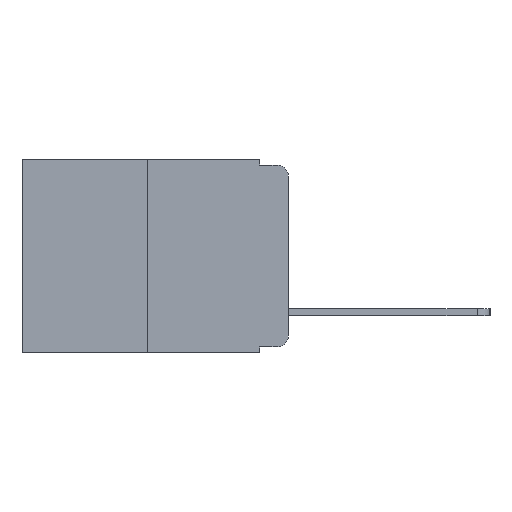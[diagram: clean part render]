
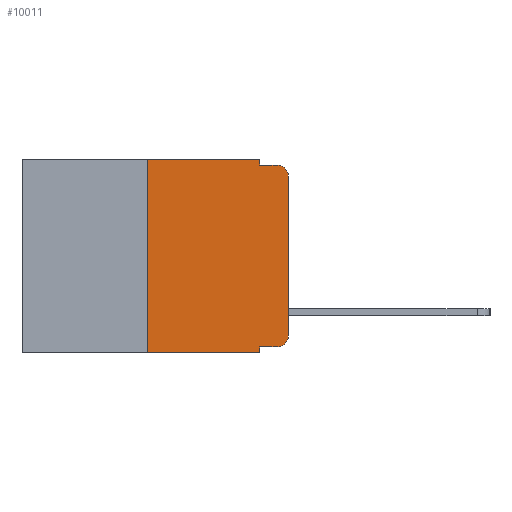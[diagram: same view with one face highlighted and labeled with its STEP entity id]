
A CAD part, left-side view. The second image highlights one B-rep face of the part: STEP entity #10011.
In plain terms, the highlighted planar face has unit normal (-1, 0, 0).
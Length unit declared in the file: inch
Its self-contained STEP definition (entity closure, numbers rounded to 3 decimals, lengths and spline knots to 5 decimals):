
#43 = ORIENTED_EDGE ( 'NONE', *, *, #9116, .T. ) ;
#146 = LINE ( 'NONE', #479, #2923 ) ;
#185 = VERTEX_POINT ( 'NONE', #4592 ) ;
#213 = VECTOR ( 'NONE', #6755, 39.37008 ) ;
#479 = CARTESIAN_POINT ( 'NONE',  ( 0., 0.25, 0. ) ) ;
#668 = CIRCLE ( 'NONE', #10164, 0.02 ) ;
#905 = VERTEX_POINT ( 'NONE', #5850 ) ;
#944 = VECTOR ( 'NONE', #1366, 39.37008 ) ;
#979 = EDGE_CURVE ( 'NONE', #8860, #3241, #3000, .T. ) ;
#1080 = CARTESIAN_POINT ( 'NONE',  ( 0., 0.25, -0.343 ) ) ;
#1091 = VERTEX_POINT ( 'NONE', #9271 ) ;
#1366 = DIRECTION ( 'NONE',  ( 0., -1., 0. ) ) ;
#1451 = EDGE_CURVE ( 'NONE', #7277, #1091, #3312, .T. ) ;
#1468 = DIRECTION ( 'NONE',  ( 0., 0., -1. ) ) ;
#1829 = EDGE_CURVE ( 'NONE', #2506, #3435, #11392, .T. ) ;
#1856 = AXIS2_PLACEMENT_3D ( 'NONE', #3533, #9774, #4496 ) ;
#1991 = CARTESIAN_POINT ( 'NONE',  ( 0., 0.051, 0. ) ) ;
#2491 = ORIENTED_EDGE ( 'NONE', *, *, #979, .T. ) ;
#2506 = VERTEX_POINT ( 'NONE', #7261 ) ;
#2726 = CIRCLE ( 'NONE', #1856, 0.02 ) ;
#2828 = ORIENTED_EDGE ( 'NONE', *, *, #1451, .F. ) ;
#2864 = EDGE_CURVE ( 'NONE', #3435, #905, #668, .T. ) ;
#2923 = VECTOR ( 'NONE', #4551, 39.37008 ) ;
#3000 = LINE ( 'NONE', #10351, #7510 ) ;
#3010 = CARTESIAN_POINT ( 'NONE',  ( 0., 0.051, 0. ) ) ;
#3162 = ORIENTED_EDGE ( 'NONE', *, *, #8479, .F. ) ;
#3241 = VERTEX_POINT ( 'NONE', #6812 ) ;
#3312 = LINE ( 'NONE', #10303, #213 ) ;
#3435 = VERTEX_POINT ( 'NONE', #4904 ) ;
#3533 = CARTESIAN_POINT ( 'NONE',  ( 0., 0.02, -0.03 ) ) ;
#3577 = DIRECTION ( 'NONE',  ( 0., 0., -1. ) ) ;
#3696 = LINE ( 'NONE', #6155, #944 ) ;
#3896 = EDGE_LOOP ( 'NONE', ( #43, #11484, #3162, #5350, #2828, #9760, #2491, #6826, #6556, #6299 ) ) ;
#4271 = VECTOR ( 'NONE', #11627, 39.37008 ) ;
#4496 = DIRECTION ( 'NONE',  ( 0., 0., -1. ) ) ;
#4505 = VECTOR ( 'NONE', #4749, 39.37008 ) ;
#4551 = DIRECTION ( 'NONE',  ( 0., 0., 1. ) ) ;
#4592 = CARTESIAN_POINT ( 'NONE',  ( 0., 0.02, -0.01 ) ) ;
#4749 = DIRECTION ( 'NONE',  ( 0., -1., 0. ) ) ;
#4904 = CARTESIAN_POINT ( 'NONE',  ( 0., 0.02, -0.333 ) ) ;
#4941 = CARTESIAN_POINT ( 'NONE',  ( 0., 0.02, -0.313 ) ) ;
#5346 = PLANE ( 'NONE',  #7872 ) ;
#5350 = ORIENTED_EDGE ( 'NONE', *, *, #11357, .F. ) ;
#5701 = VECTOR ( 'NONE', #6620, 39.37008 ) ;
#5850 = CARTESIAN_POINT ( 'NONE',  ( 0., 0., -0.313 ) ) ;
#6155 = CARTESIAN_POINT ( 'NONE',  ( 0., 0.051, -0.01 ) ) ;
#6230 = CARTESIAN_POINT ( 'NONE',  ( 0., 0.473, 0. ) ) ;
#6299 = ORIENTED_EDGE ( 'NONE', *, *, #2864, .T. ) ;
#6556 = ORIENTED_EDGE ( 'NONE', *, *, #1829, .T. ) ;
#6620 = DIRECTION ( 'NONE',  ( 0., 0., -1. ) ) ;
#6755 = DIRECTION ( 'NONE',  ( 0., -1., 0. ) ) ;
#6812 = CARTESIAN_POINT ( 'NONE',  ( 0., 0.051, -0.343 ) ) ;
#6826 = ORIENTED_EDGE ( 'NONE', *, *, #10669, .F. ) ;
#6853 = CARTESIAN_POINT ( 'NONE',  ( 0., 0.051, -0.01 ) ) ;
#7068 = DIRECTION ( 'NONE',  ( 1., 0., 0. ) ) ;
#7184 = CARTESIAN_POINT ( 'NONE',  ( 0., 0., -0.03 ) ) ;
#7245 = FACE_OUTER_BOUND ( 'NONE', #3896, .T. ) ;
#7261 = CARTESIAN_POINT ( 'NONE',  ( 0., 0.051, -0.333 ) ) ;
#7277 = VERTEX_POINT ( 'NONE', #8798 ) ;
#7439 = LINE ( 'NONE', #3010, #7748 ) ;
#7510 = VECTOR ( 'NONE', #9424, 39.37008 ) ;
#7748 = VECTOR ( 'NONE', #10187, 39.37008 ) ;
#7872 = AXIS2_PLACEMENT_3D ( 'NONE', #6230, #7068, #1468 ) ;
#8367 = CARTESIAN_POINT ( 'NONE',  ( 0., 0., 0. ) ) ;
#8388 = CARTESIAN_POINT ( 'NONE',  ( 0., 0.051, -0.333 ) ) ;
#8428 = VERTEX_POINT ( 'NONE', #6853 ) ;
#8479 = EDGE_CURVE ( 'NONE', #8428, #185, #3696, .T. ) ;
#8532 = EDGE_CURVE ( 'NONE', #8587, #185, #2726, .T. ) ;
#8587 = VERTEX_POINT ( 'NONE', #7184 ) ;
#8706 = LINE ( 'NONE', #8367, #4271 ) ;
#8798 = CARTESIAN_POINT ( 'NONE',  ( 0., 0.25, 0. ) ) ;
#8860 = VERTEX_POINT ( 'NONE', #1080 ) ;
#9116 = EDGE_CURVE ( 'NONE', #905, #8587, #8706, .T. ) ;
#9271 = CARTESIAN_POINT ( 'NONE',  ( 0., 0.051, 0. ) ) ;
#9404 = DIRECTION ( 'NONE',  ( -1., 0., 0. ) ) ;
#9424 = DIRECTION ( 'NONE',  ( 0., -1., 0. ) ) ;
#9760 = ORIENTED_EDGE ( 'NONE', *, *, #10639, .F. ) ;
#9774 = DIRECTION ( 'NONE',  ( -1., 0., 0. ) ) ;
#10011 = ADVANCED_FACE ( 'NONE', ( #7245 ), #5346, .F. ) ;
#10069 = LINE ( 'NONE', #1991, #5701 ) ;
#10164 = AXIS2_PLACEMENT_3D ( 'NONE', #4941, #9404, #3577 ) ;
#10187 = DIRECTION ( 'NONE',  ( 0., 0., -1. ) ) ;
#10303 = CARTESIAN_POINT ( 'NONE',  ( 0., 0.473, 0. ) ) ;
#10351 = CARTESIAN_POINT ( 'NONE',  ( 0., 0.473, -0.343 ) ) ;
#10639 = EDGE_CURVE ( 'NONE', #8860, #7277, #146, .T. ) ;
#10669 = EDGE_CURVE ( 'NONE', #2506, #3241, #7439, .T. ) ;
#11357 = EDGE_CURVE ( 'NONE', #1091, #8428, #10069, .T. ) ;
#11392 = LINE ( 'NONE', #8388, #4505 ) ;
#11484 = ORIENTED_EDGE ( 'NONE', *, *, #8532, .T. ) ;
#11627 = DIRECTION ( 'NONE',  ( 0., 0., 1. ) ) ;
